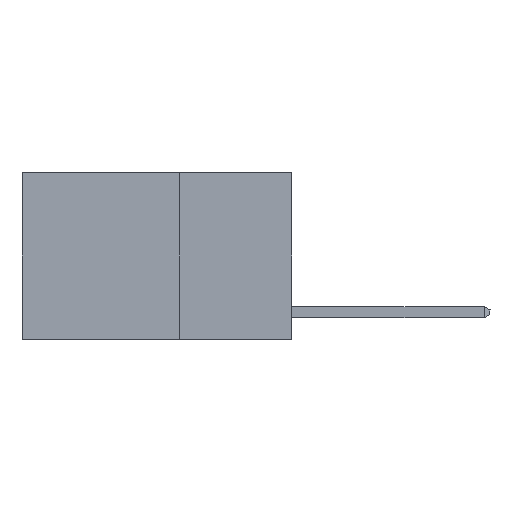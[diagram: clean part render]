
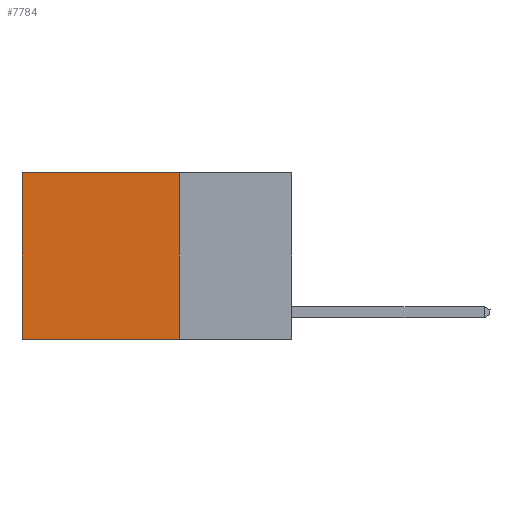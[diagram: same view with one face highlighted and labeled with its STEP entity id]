
A CAD part, left-side view. The second image highlights one B-rep face of the part: STEP entity #7784.
In plain terms, the highlighted planar face has unit normal (-1, 0, 0).
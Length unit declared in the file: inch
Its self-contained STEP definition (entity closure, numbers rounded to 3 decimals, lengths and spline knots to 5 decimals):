
#220 = AXIS2_PLACEMENT_3D ( 'NONE', #24156, #12995, #1421 ) ;
#755 = VERTEX_POINT ( 'NONE', #14086 ) ;
#788 = DIRECTION ( 'NONE',  ( 0., 0., -1. ) ) ;
#911 = LINE ( 'NONE', #10389, #9526 ) ;
#1370 = ORIENTED_EDGE ( 'NONE', *, *, #1752, .T. ) ;
#1421 = DIRECTION ( 'NONE',  ( 0., 0., -1. ) ) ;
#1752 = EDGE_CURVE ( 'NONE', #3743, #15382, #8175, .T. ) ;
#2692 = DIRECTION ( 'NONE',  ( 0., 1., 0. ) ) ;
#3743 = VERTEX_POINT ( 'NONE', #19679 ) ;
#4323 = VECTOR ( 'NONE', #4586, 39.37008 ) ;
#4586 = DIRECTION ( 'NONE',  ( 0., 0., -1. ) ) ;
#5980 = EDGE_CURVE ( 'NONE', #755, #12374, #911, .T. ) ;
#6453 = VECTOR ( 'NONE', #20437, 39.37008 ) ;
#6766 = ORIENTED_EDGE ( 'NONE', *, *, #5980, .F. ) ;
#6911 = EDGE_LOOP ( 'NONE', ( #1370, #20483, #6766, #10100 ) ) ;
#7617 = CARTESIAN_POINT ( 'NONE',  ( 0.2625, 0.25, -0.37 ) ) ;
#7784 = ADVANCED_FACE ( 'NONE', ( #8844 ), #20576, .F. ) ;
#8175 = LINE ( 'NONE', #11213, #4323 ) ;
#8844 = FACE_OUTER_BOUND ( 'NONE', #6911, .T. ) ;
#9526 = VECTOR ( 'NONE', #788, 39.37008 ) ;
#9845 = CARTESIAN_POINT ( 'NONE',  ( 0.2625, 0.25, -0.37 ) ) ;
#10100 = ORIENTED_EDGE ( 'NONE', *, *, #14056, .T. ) ;
#10389 = CARTESIAN_POINT ( 'NONE',  ( 0.2625, 0.25, 0. ) ) ;
#11213 = CARTESIAN_POINT ( 'NONE',  ( 0.2625, 0.6, 0. ) ) ;
#12289 = EDGE_CURVE ( 'NONE', #12374, #15382, #14853, .T. ) ;
#12374 = VERTEX_POINT ( 'NONE', #9845 ) ;
#12995 = DIRECTION ( 'NONE',  ( 1., 0., 0. ) ) ;
#14056 = EDGE_CURVE ( 'NONE', #755, #3743, #21875, .T. ) ;
#14086 = CARTESIAN_POINT ( 'NONE',  ( 0.2625, 0.25, 0. ) ) ;
#14853 = LINE ( 'NONE', #7617, #21691 ) ;
#15382 = VERTEX_POINT ( 'NONE', #19609 ) ;
#19609 = CARTESIAN_POINT ( 'NONE',  ( 0.2625, 0.6, -0.37 ) ) ;
#19679 = CARTESIAN_POINT ( 'NONE',  ( 0.2625, 0.6, 0. ) ) ;
#20437 = DIRECTION ( 'NONE',  ( 0., 1., 0. ) ) ;
#20483 = ORIENTED_EDGE ( 'NONE', *, *, #12289, .F. ) ;
#20576 = PLANE ( 'NONE',  #220 ) ;
#21691 = VECTOR ( 'NONE', #2692, 39.37008 ) ;
#21875 = LINE ( 'NONE', #22093, #6453 ) ;
#22093 = CARTESIAN_POINT ( 'NONE',  ( 0.2625, 0.25, 0. ) ) ;
#24156 = CARTESIAN_POINT ( 'NONE',  ( 0.2625, 0.25, 0. ) ) ;
